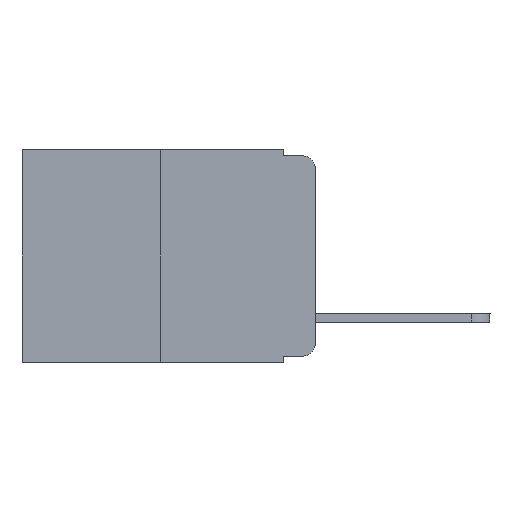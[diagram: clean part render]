
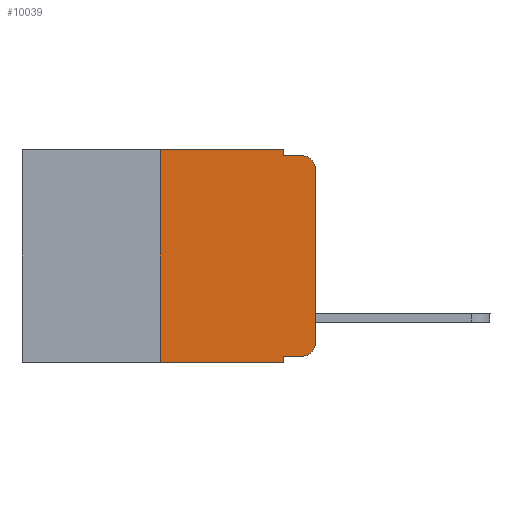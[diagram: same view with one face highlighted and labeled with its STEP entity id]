
A CAD part, left-side view. The second image highlights one B-rep face of the part: STEP entity #10039.
In plain terms, the highlighted planar face has unit normal (-1, 0, 0).
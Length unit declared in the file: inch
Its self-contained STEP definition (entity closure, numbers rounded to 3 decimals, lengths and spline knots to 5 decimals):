
#764 = VERTEX_POINT ( 'NONE', #15335 ) ;
#1292 = VERTEX_POINT ( 'NONE', #12526 ) ;
#1376 = ORIENTED_EDGE ( 'NONE', *, *, #16671, .T. ) ;
#1425 = ORIENTED_EDGE ( 'NONE', *, *, #9901, .F. ) ;
#1542 = EDGE_CURVE ( 'NONE', #764, #4693, #5637, .T. ) ;
#1563 = EDGE_CURVE ( 'NONE', #19084, #14235, #13780, .T. ) ;
#1606 = ORIENTED_EDGE ( 'NONE', *, *, #1542, .T. ) ;
#1739 = VERTEX_POINT ( 'NONE', #7608 ) ;
#1906 = VECTOR ( 'NONE', #16830, 39.37008 ) ;
#3915 = ORIENTED_EDGE ( 'NONE', *, *, #11624, .F. ) ;
#3960 = LINE ( 'NONE', #10427, #19603 ) ;
#4196 = EDGE_CURVE ( 'NONE', #18033, #10812, #10765, .T. ) ;
#4293 = PLANE ( 'NONE',  #16839 ) ;
#4587 = ORIENTED_EDGE ( 'NONE', *, *, #7402, .T. ) ;
#4607 = DIRECTION ( 'NONE',  ( 1., 0., 0. ) ) ;
#4615 = CARTESIAN_POINT ( 'NONE',  ( 0., 0.051, -0.333 ) ) ;
#4639 = CARTESIAN_POINT ( 'NONE',  ( 0., 0.02, -0.03 ) ) ;
#4693 = VERTEX_POINT ( 'NONE', #15936 ) ;
#5157 = ORIENTED_EDGE ( 'NONE', *, *, #1563, .F. ) ;
#5396 = DIRECTION ( 'NONE',  ( 0., 0., 1. ) ) ;
#5637 = CIRCLE ( 'NONE', #19171, 0.02 ) ;
#5794 = CARTESIAN_POINT ( 'NONE',  ( 0., 0.051, 0. ) ) ;
#6213 = FACE_OUTER_BOUND ( 'NONE', #13477, .T. ) ;
#6323 = CARTESIAN_POINT ( 'NONE',  ( 0., 0.473, 0. ) ) ;
#7203 = CARTESIAN_POINT ( 'NONE',  ( 0., 0.051, -0.01 ) ) ;
#7402 = EDGE_CURVE ( 'NONE', #4693, #13386, #12670, .T. ) ;
#7412 = DIRECTION ( 'NONE',  ( 0., 0., -1. ) ) ;
#7608 = CARTESIAN_POINT ( 'NONE',  ( 0., 0.051, -0.333 ) ) ;
#8026 = LINE ( 'NONE', #20859, #8936 ) ;
#8114 = DIRECTION ( 'NONE',  ( 0., -1., 0. ) ) ;
#8936 = VECTOR ( 'NONE', #20437, 39.37008 ) ;
#9028 = VECTOR ( 'NONE', #15054, 39.37008 ) ;
#9396 = CARTESIAN_POINT ( 'NONE',  ( 0., 0., 0. ) ) ;
#9554 = CARTESIAN_POINT ( 'NONE',  ( 0., 0., -0.03 ) ) ;
#9738 = DIRECTION ( 'NONE',  ( 0., 0., -1. ) ) ;
#9802 = LINE ( 'NONE', #11507, #13016 ) ;
#9901 = EDGE_CURVE ( 'NONE', #1739, #16507, #10457, .T. ) ;
#10039 = ADVANCED_FACE ( 'NONE', ( #6213 ), #4293, .F. ) ;
#10273 = DIRECTION ( 'NONE',  ( -1., 0., 0. ) ) ;
#10427 = CARTESIAN_POINT ( 'NONE',  ( 0., 0.051, 0. ) ) ;
#10457 = LINE ( 'NONE', #5794, #1906 ) ;
#10765 = LINE ( 'NONE', #12574, #19849 ) ;
#10809 = AXIS2_PLACEMENT_3D ( 'NONE', #4639, #17692, #9738 ) ;
#10812 = VERTEX_POINT ( 'NONE', #16674 ) ;
#10917 = ORIENTED_EDGE ( 'NONE', *, *, #16055, .F. ) ;
#11163 = VECTOR ( 'NONE', #20735, 39.37008 ) ;
#11507 = CARTESIAN_POINT ( 'NONE',  ( 0., 0.473, -0.343 ) ) ;
#11624 = EDGE_CURVE ( 'NONE', #1292, #19084, #3960, .T. ) ;
#11711 = VECTOR ( 'NONE', #14282, 39.37008 ) ;
#12123 = EDGE_CURVE ( 'NONE', #13386, #14235, #15497, .T. ) ;
#12227 = CARTESIAN_POINT ( 'NONE',  ( 0., 0.25, -0.343 ) ) ;
#12526 = CARTESIAN_POINT ( 'NONE',  ( 0., 0.051, 0. ) ) ;
#12574 = CARTESIAN_POINT ( 'NONE',  ( 0., 0.25, 0. ) ) ;
#12670 = LINE ( 'NONE', #9396, #11163 ) ;
#13016 = VECTOR ( 'NONE', #8114, 39.37008 ) ;
#13386 = VERTEX_POINT ( 'NONE', #9554 ) ;
#13477 = EDGE_LOOP ( 'NONE', ( #4587, #18584, #5157, #3915, #10917, #17333, #1376, #1425, #18298, #1606 ) ) ;
#13724 = DIRECTION ( 'NONE',  ( 0., 0., -1. ) ) ;
#13780 = LINE ( 'NONE', #7203, #9028 ) ;
#13867 = CARTESIAN_POINT ( 'NONE',  ( 0., 0.051, -0.01 ) ) ;
#14160 = CARTESIAN_POINT ( 'NONE',  ( 0., 0.051, -0.343 ) ) ;
#14235 = VERTEX_POINT ( 'NONE', #14459 ) ;
#14282 = DIRECTION ( 'NONE',  ( 0., -1., 0. ) ) ;
#14459 = CARTESIAN_POINT ( 'NONE',  ( 0., 0.02, -0.01 ) ) ;
#15054 = DIRECTION ( 'NONE',  ( 0., -1., 0. ) ) ;
#15335 = CARTESIAN_POINT ( 'NONE',  ( 0., 0.02, -0.333 ) ) ;
#15497 = CIRCLE ( 'NONE', #10809, 0.02 ) ;
#15875 = LINE ( 'NONE', #4615, #11711 ) ;
#15936 = CARTESIAN_POINT ( 'NONE',  ( 0., 0., -0.313 ) ) ;
#16055 = EDGE_CURVE ( 'NONE', #10812, #1292, #8026, .T. ) ;
#16507 = VERTEX_POINT ( 'NONE', #14160 ) ;
#16648 = CARTESIAN_POINT ( 'NONE',  ( 0., 0.02, -0.313 ) ) ;
#16671 = EDGE_CURVE ( 'NONE', #18033, #16507, #9802, .T. ) ;
#16674 = CARTESIAN_POINT ( 'NONE',  ( 0., 0.25, 0. ) ) ;
#16830 = DIRECTION ( 'NONE',  ( 0., 0., -1. ) ) ;
#16839 = AXIS2_PLACEMENT_3D ( 'NONE', #6323, #4607, #20533 ) ;
#17333 = ORIENTED_EDGE ( 'NONE', *, *, #4196, .F. ) ;
#17692 = DIRECTION ( 'NONE',  ( -1., 0., 0. ) ) ;
#18033 = VERTEX_POINT ( 'NONE', #12227 ) ;
#18298 = ORIENTED_EDGE ( 'NONE', *, *, #19168, .T. ) ;
#18584 = ORIENTED_EDGE ( 'NONE', *, *, #12123, .T. ) ;
#19084 = VERTEX_POINT ( 'NONE', #13867 ) ;
#19168 = EDGE_CURVE ( 'NONE', #1739, #764, #15875, .T. ) ;
#19171 = AXIS2_PLACEMENT_3D ( 'NONE', #16648, #10273, #7412 ) ;
#19603 = VECTOR ( 'NONE', #13724, 39.37008 ) ;
#19849 = VECTOR ( 'NONE', #5396, 39.37008 ) ;
#20437 = DIRECTION ( 'NONE',  ( 0., -1., 0. ) ) ;
#20533 = DIRECTION ( 'NONE',  ( 0., 0., -1. ) ) ;
#20735 = DIRECTION ( 'NONE',  ( 0., 0., 1. ) ) ;
#20859 = CARTESIAN_POINT ( 'NONE',  ( 0., 0.473, 0. ) ) ;
